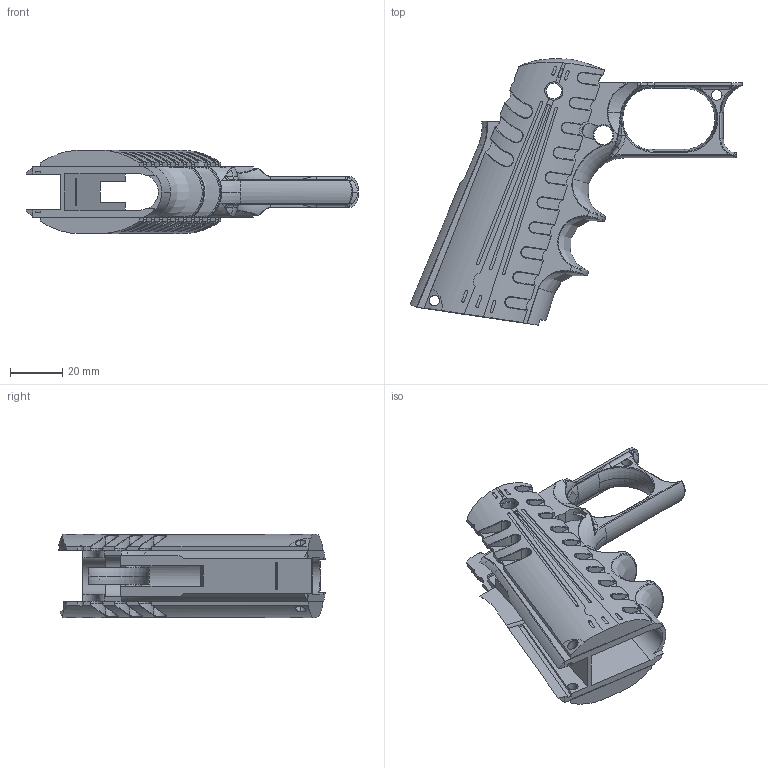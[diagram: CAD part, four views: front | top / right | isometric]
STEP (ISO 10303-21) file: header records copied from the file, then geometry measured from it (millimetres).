
FILE_DESCRIPTION (( 'STEP AP214' ), '1' );
FILE_NAME ('Grip_Single.STEP', '2013-07-30T15:11:52', ( 'Asher' ), ( '' ), 'SwSTEP 2.0', 'SolidWorks 2013', '' );
FILE_SCHEMA (( 'AUTOMOTIVE_DESIGN' ));
Length unit declared in the file: millimetre
Products named in the file (1): Grip_Single
Bounding box: 127.38 x 102.24 x 32.05 mm (x, y, z)
Volume: 61663.1 mm3; surface area: 31519 mm2
Topology: 1 solids, 3 shells, 848 faces, 2280 edges, 1442 vertices
Faces by surface type: plane 330, cylinder 260, bspline 207, torus 47, sphere 4
Entity records: 35916 total; most frequent: CARTESIAN_POINT 16242, ORIENTED_EDGE 4552, DIRECTION 3291, EDGE_CURVE 2276, VERTEX_POINT 1442, AXIS2_PLACEMENT_3D 1183, LINE 925, VECTOR 925
